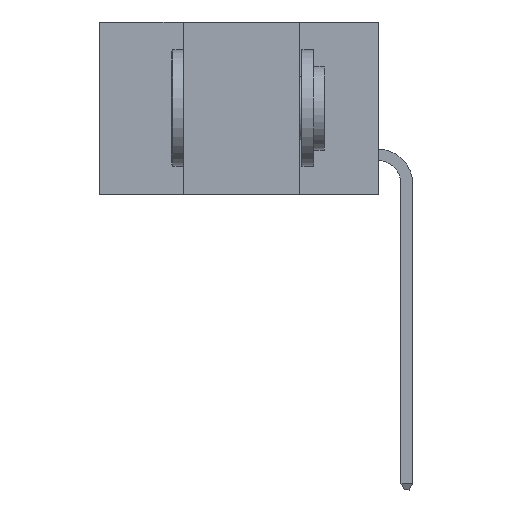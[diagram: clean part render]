
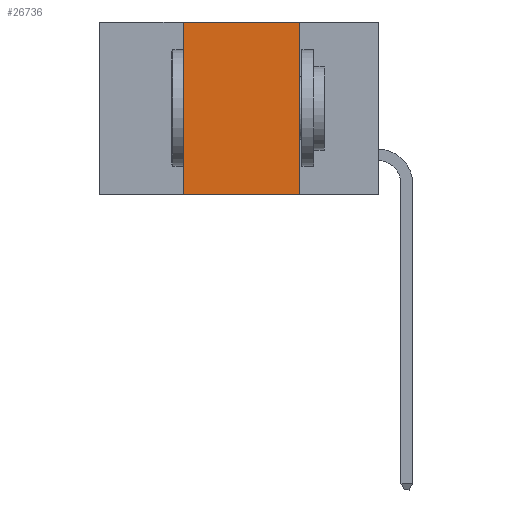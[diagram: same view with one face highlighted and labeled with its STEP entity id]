
A CAD part, left-side view. The second image highlights one B-rep face of the part: STEP entity #26736.
In plain terms, the highlighted planar face has unit normal (-1, 0, 0).
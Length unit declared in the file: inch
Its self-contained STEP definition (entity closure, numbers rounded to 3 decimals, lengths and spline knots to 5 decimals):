
#1217 = VERTEX_POINT ( 'NONE', #11432 ) ;
#1600 = LINE ( 'NONE', #16296, #15169 ) ;
#2038 = VERTEX_POINT ( 'NONE', #31613 ) ;
#2846 = EDGE_CURVE ( 'NONE', #8870, #30221, #26552, .T. ) ;
#4051 = FACE_OUTER_BOUND ( 'NONE', #30761, .T. ) ;
#4072 = CARTESIAN_POINT ( 'NONE',  ( 0., 0.6, 0. ) ) ;
#5206 = AXIS2_PLACEMENT_3D ( 'NONE', #4072, #21847, #6656 ) ;
#6321 = DIRECTION ( 'NONE',  ( 0., 0., 1. ) ) ;
#6656 = DIRECTION ( 'NONE',  ( 0., 0., -1. ) ) ;
#7118 = VECTOR ( 'NONE', #25768, 39.37008 ) ;
#8213 = VECTOR ( 'NONE', #12031, 39.37008 ) ;
#8693 = ORIENTED_EDGE ( 'NONE', *, *, #27263, .T. ) ;
#8870 = VERTEX_POINT ( 'NONE', #28028 ) ;
#11148 = VECTOR ( 'NONE', #6321, 39.37008 ) ;
#11432 = CARTESIAN_POINT ( 'NONE',  ( 0., 0.42, -0.37 ) ) ;
#11696 = CARTESIAN_POINT ( 'NONE',  ( 0., 0.17, -0.37 ) ) ;
#12031 = DIRECTION ( 'NONE',  ( 0., -1., 0. ) ) ;
#12687 = ORIENTED_EDGE ( 'NONE', *, *, #24593, .F. ) ;
#12757 = LINE ( 'NONE', #23950, #11148 ) ;
#14981 = LINE ( 'NONE', #19528, #8213 ) ;
#15169 = VECTOR ( 'NONE', #18824, 39.37008 ) ;
#16296 = CARTESIAN_POINT ( 'NONE',  ( 0., 0.6, -0.37 ) ) ;
#18824 = DIRECTION ( 'NONE',  ( 0., -1., 0. ) ) ;
#19528 = CARTESIAN_POINT ( 'NONE',  ( 0., 0.6, 0. ) ) ;
#19819 = ORIENTED_EDGE ( 'NONE', *, *, #32197, .F. ) ;
#21750 = PLANE ( 'NONE',  #5206 ) ;
#21847 = DIRECTION ( 'NONE',  ( 1., 0., 0. ) ) ;
#23950 = CARTESIAN_POINT ( 'NONE',  ( 0., 0.42, 0. ) ) ;
#24593 = EDGE_CURVE ( 'NONE', #2038, #8870, #14981, .T. ) ;
#25768 = DIRECTION ( 'NONE',  ( 0., 0., -1. ) ) ;
#26552 = LINE ( 'NONE', #27866, #7118 ) ;
#26736 = ADVANCED_FACE ( 'NONE', ( #4051 ), #21750, .F. ) ;
#27263 = EDGE_CURVE ( 'NONE', #1217, #30221, #1600, .T. ) ;
#27866 = CARTESIAN_POINT ( 'NONE',  ( 0., 0.17, 0. ) ) ;
#28028 = CARTESIAN_POINT ( 'NONE',  ( 0., 0.17, 0. ) ) ;
#30221 = VERTEX_POINT ( 'NONE', #11696 ) ;
#30761 = EDGE_LOOP ( 'NONE', ( #31893, #12687, #19819, #8693 ) ) ;
#31613 = CARTESIAN_POINT ( 'NONE',  ( 0., 0.42, 0. ) ) ;
#31893 = ORIENTED_EDGE ( 'NONE', *, *, #2846, .F. ) ;
#32197 = EDGE_CURVE ( 'NONE', #1217, #2038, #12757, .T. ) ;
